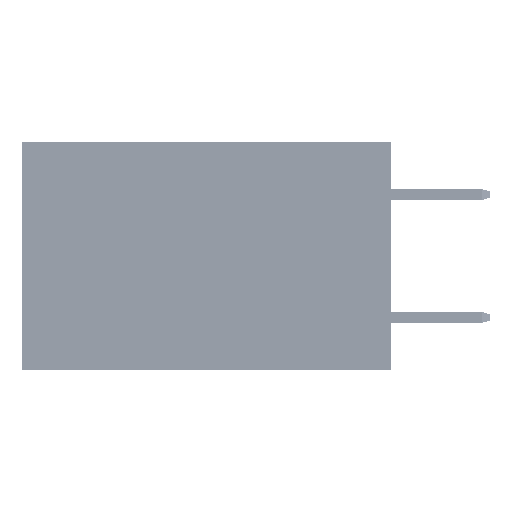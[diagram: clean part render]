
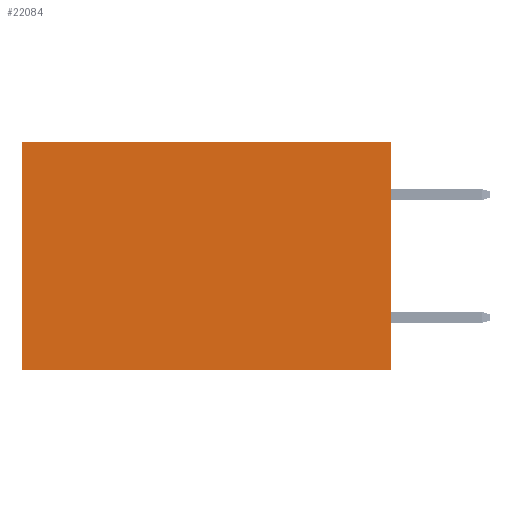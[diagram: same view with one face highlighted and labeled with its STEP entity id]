
A CAD part, left-side view. The second image highlights one B-rep face of the part: STEP entity #22084.
In plain terms, the highlighted planar face has unit normal (-1, 0, 0).
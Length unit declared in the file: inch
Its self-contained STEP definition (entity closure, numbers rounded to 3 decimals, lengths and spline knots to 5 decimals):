
#363 = DIRECTION ( 'NONE',  ( 0., 0., -1. ) ) ;
#1090 = DIRECTION ( 'NONE',  ( 0., 0., -1. ) ) ;
#2074 = DIRECTION ( 'NONE',  ( 0., 1., 0. ) ) ;
#3075 = FACE_OUTER_BOUND ( 'NONE', #25390, .T. ) ;
#3165 = ORIENTED_EDGE ( 'NONE', *, *, #22938, .T. ) ;
#3880 = EDGE_CURVE ( 'NONE', #7933, #16569, #40245, .T. ) ;
#3939 = CARTESIAN_POINT ( 'NONE',  ( 0.2875, 0.6, 0. ) ) ;
#4200 = ORIENTED_EDGE ( 'NONE', *, *, #3880, .T. ) ;
#5349 = EDGE_CURVE ( 'NONE', #7933, #36461, #11080, .T. ) ;
#5640 = CARTESIAN_POINT ( 'NONE',  ( 0.2875, 0.6, 0. ) ) ;
#7933 = VERTEX_POINT ( 'NONE', #48454 ) ;
#7980 = EDGE_CURVE ( 'NONE', #36461, #18317, #34480, .T. ) ;
#10225 = CARTESIAN_POINT ( 'NONE',  ( 0.2875, 0., 0. ) ) ;
#10775 = CARTESIAN_POINT ( 'NONE',  ( 0.2875, 0., 0. ) ) ;
#11080 = LINE ( 'NONE', #10775, #19926 ) ;
#14024 = DIRECTION ( 'NONE',  ( 0., 0., -1. ) ) ;
#16055 = VECTOR ( 'NONE', #2074, 39.37008 ) ;
#16569 = VERTEX_POINT ( 'NONE', #5640 ) ;
#17741 = CARTESIAN_POINT ( 'NONE',  ( 0.2875, 0.6, -0.37 ) ) ;
#18317 = VERTEX_POINT ( 'NONE', #17741 ) ;
#19926 = VECTOR ( 'NONE', #363, 39.37008 ) ;
#20091 = LINE ( 'NONE', #3939, #37889 ) ;
#20338 = CARTESIAN_POINT ( 'NONE',  ( 0.2875, 0., 0. ) ) ;
#20678 = VECTOR ( 'NONE', #42204, 39.37008 ) ;
#21995 = AXIS2_PLACEMENT_3D ( 'NONE', #10225, #40702, #14024 ) ;
#22084 = ADVANCED_FACE ( 'NONE', ( #3075 ), #40872, .F. ) ;
#22938 = EDGE_CURVE ( 'NONE', #16569, #18317, #20091, .T. ) ;
#25390 = EDGE_LOOP ( 'NONE', ( #3165, #41141, #45583, #4200 ) ) ;
#34480 = LINE ( 'NONE', #47394, #16055 ) ;
#36461 = VERTEX_POINT ( 'NONE', #41818 ) ;
#37889 = VECTOR ( 'NONE', #1090, 39.37008 ) ;
#40245 = LINE ( 'NONE', #20338, #20678 ) ;
#40702 = DIRECTION ( 'NONE',  ( 1., 0., 0. ) ) ;
#40872 = PLANE ( 'NONE',  #21995 ) ;
#41141 = ORIENTED_EDGE ( 'NONE', *, *, #7980, .F. ) ;
#41818 = CARTESIAN_POINT ( 'NONE',  ( 0.2875, 0., -0.37 ) ) ;
#42204 = DIRECTION ( 'NONE',  ( 0., 1., 0. ) ) ;
#45583 = ORIENTED_EDGE ( 'NONE', *, *, #5349, .F. ) ;
#47394 = CARTESIAN_POINT ( 'NONE',  ( 0.2875, 0., -0.37 ) ) ;
#48454 = CARTESIAN_POINT ( 'NONE',  ( 0.2875, 0., 0. ) ) ;
